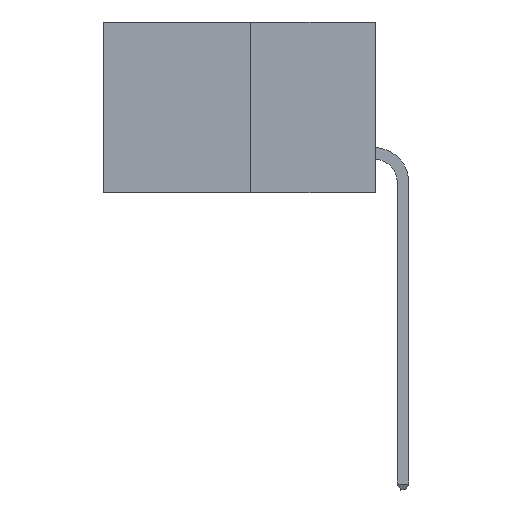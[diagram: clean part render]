
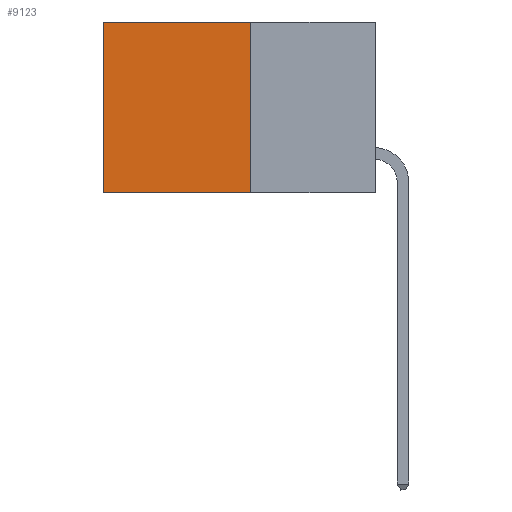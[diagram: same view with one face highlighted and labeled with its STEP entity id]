
A CAD part, left-side view. The second image highlights one B-rep face of the part: STEP entity #9123.
In plain terms, the highlighted planar face has unit normal (-1, 0, 0).
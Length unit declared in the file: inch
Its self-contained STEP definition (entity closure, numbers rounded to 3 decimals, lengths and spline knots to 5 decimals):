
#32 = VECTOR ( 'NONE', #243, 39.37008 ) ;
#243 = DIRECTION ( 'NONE',  ( 0., 0., -1. ) ) ;
#1374 = VERTEX_POINT ( 'NONE', #13263 ) ;
#1816 = ORIENTED_EDGE ( 'NONE', *, *, #11538, .F. ) ;
#2364 = DIRECTION ( 'NONE',  ( 0., 0., -1. ) ) ;
#2436 = LINE ( 'NONE', #23042, #14154 ) ;
#2509 = VERTEX_POINT ( 'NONE', #8985 ) ;
#3319 = VERTEX_POINT ( 'NONE', #22449 ) ;
#3412 = AXIS2_PLACEMENT_3D ( 'NONE', #28659, #21917, #21911 ) ;
#4083 = DIRECTION ( 'NONE',  ( 0., 1., 0. ) ) ;
#5952 = EDGE_LOOP ( 'NONE', ( #21896, #21152, #1816, #11196 ) ) ;
#6807 = CARTESIAN_POINT ( 'NONE',  ( 0.277, 0.27, -0.37 ) ) ;
#6947 = EDGE_CURVE ( 'NONE', #1374, #2509, #2436, .T. ) ;
#8985 = CARTESIAN_POINT ( 'NONE',  ( 0.277, 0.59, 0. ) ) ;
#9123 = ADVANCED_FACE ( 'NONE', ( #14420 ), #26402, .F. ) ;
#10967 = VERTEX_POINT ( 'NONE', #6807 ) ;
#11196 = ORIENTED_EDGE ( 'NONE', *, *, #6947, .T. ) ;
#11538 = EDGE_CURVE ( 'NONE', #1374, #10967, #12556, .T. ) ;
#11693 = CARTESIAN_POINT ( 'NONE',  ( 0.277, 0.27, -0.37 ) ) ;
#12556 = LINE ( 'NONE', #11693, #32 ) ;
#13263 = CARTESIAN_POINT ( 'NONE',  ( 0.277, 0.27, 0. ) ) ;
#13329 = VECTOR ( 'NONE', #14548, 39.37008 ) ;
#14071 = LINE ( 'NONE', #21337, #13329 ) ;
#14154 = VECTOR ( 'NONE', #4083, 39.37008 ) ;
#14420 = FACE_OUTER_BOUND ( 'NONE', #5952, .T. ) ;
#14548 = DIRECTION ( 'NONE',  ( 0., 1., 0. ) ) ;
#19851 = VECTOR ( 'NONE', #2364, 39.37008 ) ;
#20840 = CARTESIAN_POINT ( 'NONE',  ( 0.277, 0.59, -0.37 ) ) ;
#21152 = ORIENTED_EDGE ( 'NONE', *, *, #29309, .F. ) ;
#21337 = CARTESIAN_POINT ( 'NONE',  ( 0.277, 0.27, -0.37 ) ) ;
#21896 = ORIENTED_EDGE ( 'NONE', *, *, #24476, .T. ) ;
#21911 = DIRECTION ( 'NONE',  ( 0., 0., -1. ) ) ;
#21917 = DIRECTION ( 'NONE',  ( 1., 0., 0. ) ) ;
#22449 = CARTESIAN_POINT ( 'NONE',  ( 0.277, 0.59, -0.37 ) ) ;
#23042 = CARTESIAN_POINT ( 'NONE',  ( 0.277, 0.27, 0. ) ) ;
#24476 = EDGE_CURVE ( 'NONE', #2509, #3319, #25907, .T. ) ;
#25907 = LINE ( 'NONE', #20840, #19851 ) ;
#26402 = PLANE ( 'NONE',  #3412 ) ;
#28659 = CARTESIAN_POINT ( 'NONE',  ( 0.277, 0.27, -0.37 ) ) ;
#29309 = EDGE_CURVE ( 'NONE', #10967, #3319, #14071, .T. ) ;
